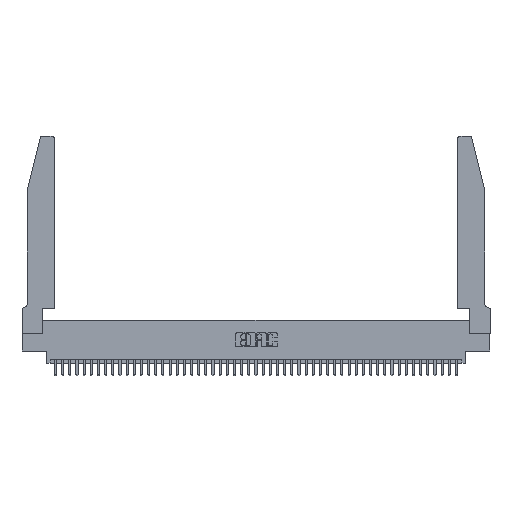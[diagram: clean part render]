
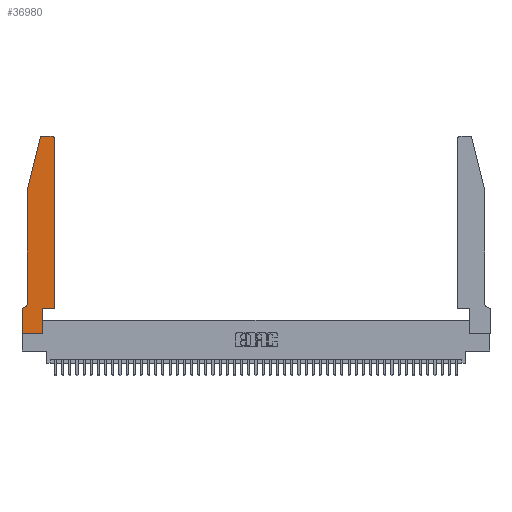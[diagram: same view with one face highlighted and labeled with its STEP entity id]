
A CAD part, top view. The second image highlights one B-rep face of the part: STEP entity #36980.
In plain terms, the highlighted planar face has unit normal (0, 0, 1).
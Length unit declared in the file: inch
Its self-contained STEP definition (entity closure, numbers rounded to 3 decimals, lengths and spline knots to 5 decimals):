
#577 = VERTEX_POINT ( 'NONE', #38761 ) ;
#1104 = EDGE_CURVE ( 'NONE', #37065, #6819, #38696, .T. ) ;
#2470 = ORIENTED_EDGE ( 'NONE', *, *, #8268, .T. ) ;
#2622 = ORIENTED_EDGE ( 'NONE', *, *, #1104, .T. ) ;
#2773 = CARTESIAN_POINT ( 'NONE',  ( 0.25487, 2.72718, 0.37 ) ) ;
#3654 = FACE_OUTER_BOUND ( 'NONE', #13725, .T. ) ;
#4051 = CARTESIAN_POINT ( 'NONE',  ( 0.4505, 2.72, 0.37 ) ) ;
#4359 = PLANE ( 'NONE',  #20301 ) ;
#4523 = CARTESIAN_POINT ( 'NONE',  ( 0., 0.35, 0.37 ) ) ;
#4540 = VERTEX_POINT ( 'NONE', #16303 ) ;
#5442 = CARTESIAN_POINT ( 'NONE',  ( 0., 0., 0.37 ) ) ;
#5513 = LINE ( 'NONE', #27199, #11266 ) ;
#6732 = ORIENTED_EDGE ( 'NONE', *, *, #28557, .T. ) ;
#6754 = ORIENTED_EDGE ( 'NONE', *, *, #29712, .T. ) ;
#6819 = VERTEX_POINT ( 'NONE', #4051 ) ;
#7427 = VECTOR ( 'NONE', #44058, 39.37008 ) ;
#7572 = CARTESIAN_POINT ( 'NONE',  ( 0., 0., 0.37 ) ) ;
#7674 = VECTOR ( 'NONE', #18357, 39.37008 ) ;
#7821 = VECTOR ( 'NONE', #46020, 39.37008 ) ;
#7872 = VECTOR ( 'NONE', #15080, 39.37008 ) ;
#7947 = EDGE_CURVE ( 'NONE', #42472, #577, #43633, .T. ) ;
#8268 = EDGE_CURVE ( 'NONE', #4540, #11509, #31490, .T. ) ;
#8366 = VECTOR ( 'NONE', #32434, 39.37008 ) ;
#8466 = AXIS2_PLACEMENT_3D ( 'NONE', #10056, #24803, #26848 ) ;
#8479 = ORIENTED_EDGE ( 'NONE', *, *, #18645, .T. ) ;
#8747 = CARTESIAN_POINT ( 'NONE',  ( 0.4205, 2.72, 0.37 ) ) ;
#8918 = DIRECTION ( 'NONE',  ( 0., 0., 1. ) ) ;
#9044 = CARTESIAN_POINT ( 'NONE',  ( 0.4505, 0.35, 0.37 ) ) ;
#9473 = CARTESIAN_POINT ( 'NONE',  ( 0.0055, 0.42, 0.37 ) ) ;
#9497 = CARTESIAN_POINT ( 'NONE',  ( 0.2865, 0.35, 0.37 ) ) ;
#9647 = VECTOR ( 'NONE', #31269, 39.37008 ) ;
#9794 = VERTEX_POINT ( 'NONE', #41018 ) ;
#10056 = CARTESIAN_POINT ( 'NONE',  ( 0.284, 2.72, 0.37 ) ) ;
#10927 = EDGE_CURVE ( 'NONE', #577, #16014, #38673, .T. ) ;
#11266 = VECTOR ( 'NONE', #34308, 39.37008 ) ;
#11356 = VERTEX_POINT ( 'NONE', #34246 ) ;
#11509 = VERTEX_POINT ( 'NONE', #7572 ) ;
#11612 = CARTESIAN_POINT ( 'NONE',  ( 0.4205, 2.75, 0.37 ) ) ;
#11989 = LINE ( 'NONE', #15483, #24116 ) ;
#12301 = DIRECTION ( 'NONE',  ( 1., 0., 0. ) ) ;
#12440 = DIRECTION ( 'NONE',  ( 0., 1., 0. ) ) ;
#13406 = CARTESIAN_POINT ( 'NONE',  ( 0.2865, 0.35, 0.37 ) ) ;
#13725 = EDGE_LOOP ( 'NONE', ( #19344, #43618, #42547, #18176, #6732, #8479, #2470, #25183, #6754, #41848, #2622, #16489 ) ) ;
#14187 = VERTEX_POINT ( 'NONE', #32328 ) ;
#14326 = CARTESIAN_POINT ( 'NONE',  ( 0., 0., 0.37 ) ) ;
#15080 = DIRECTION ( 'NONE',  ( -1., 0., 0. ) ) ;
#15483 = CARTESIAN_POINT ( 'NONE',  ( 0.4505, 0.35, 0.37 ) ) ;
#16014 = VERTEX_POINT ( 'NONE', #2773 ) ;
#16086 = LINE ( 'NONE', #25350, #7427 ) ;
#16303 = CARTESIAN_POINT ( 'NONE',  ( 0., 0.35, 0.37 ) ) ;
#16489 = ORIENTED_EDGE ( 'NONE', *, *, #43840, .T. ) ;
#16818 = VECTOR ( 'NONE', #12440, 39.37008 ) ;
#18176 = ORIENTED_EDGE ( 'NONE', *, *, #28774, .T. ) ;
#18357 = DIRECTION ( 'NONE',  ( 1., 0., 0. ) ) ;
#18645 = EDGE_CURVE ( 'NONE', #11356, #4540, #5513, .T. ) ;
#19344 = ORIENTED_EDGE ( 'NONE', *, *, #7947, .T. ) ;
#19802 = EDGE_CURVE ( 'NONE', #16014, #9794, #40128, .T. ) ;
#20301 = AXIS2_PLACEMENT_3D ( 'NONE', #4523, #37547, #30610 ) ;
#23054 = DIRECTION ( 'NONE',  ( 1., 0., 0. ) ) ;
#24058 = EDGE_CURVE ( 'NONE', #45467, #37065, #11989, .T. ) ;
#24116 = VECTOR ( 'NONE', #23054, 39.37008 ) ;
#24803 = DIRECTION ( 'NONE',  ( 0., 0., 1. ) ) ;
#25183 = ORIENTED_EDGE ( 'NONE', *, *, #32283, .T. ) ;
#25350 = CARTESIAN_POINT ( 'NONE',  ( 0.0755, 2., 0.37 ) ) ;
#26848 = DIRECTION ( 'NONE',  ( 1., 0., 0. ) ) ;
#27199 = CARTESIAN_POINT ( 'NONE',  ( 0.0755, 0.35, 0.37 ) ) ;
#27528 = AXIS2_PLACEMENT_3D ( 'NONE', #8747, #8918, #12301 ) ;
#28557 = EDGE_CURVE ( 'NONE', #14187, #11356, #39166, .T. ) ;
#28774 = EDGE_CURVE ( 'NONE', #9794, #14187, #16086, .T. ) ;
#29712 = EDGE_CURVE ( 'NONE', #38966, #45467, #36178, .T. ) ;
#30610 = DIRECTION ( 'NONE',  ( 1., 0., 0. ) ) ;
#31046 = DIRECTION ( 'NONE',  ( 0., 0., -1. ) ) ;
#31269 = DIRECTION ( 'NONE',  ( 0., 1., 0. ) ) ;
#31281 = CARTESIAN_POINT ( 'NONE',  ( 0.4505, 0.35, 0.37 ) ) ;
#31490 = LINE ( 'NONE', #5442, #7821 ) ;
#32283 = EDGE_CURVE ( 'NONE', #11509, #38966, #39449, .T. ) ;
#32328 = CARTESIAN_POINT ( 'NONE',  ( 0.0755, 0.42, 0.37 ) ) ;
#32434 = DIRECTION ( 'NONE',  ( -0.239, -0.971, 0. ) ) ;
#34246 = CARTESIAN_POINT ( 'NONE',  ( 0.0055, 0.35, 0.37 ) ) ;
#34308 = DIRECTION ( 'NONE',  ( -1., 0., 0. ) ) ;
#34810 = CARTESIAN_POINT ( 'NONE',  ( 0.2865, 0., 0.37 ) ) ;
#35246 = DIRECTION ( 'NONE',  ( -1., 0., 0. ) ) ;
#36178 = LINE ( 'NONE', #13406, #9647 ) ;
#36980 = ADVANCED_FACE ( 'NONE', ( #3654 ), #4359, .T. ) ;
#37065 = VERTEX_POINT ( 'NONE', #9044 ) ;
#37547 = DIRECTION ( 'NONE',  ( 0., 0., 1. ) ) ;
#38100 = CIRCLE ( 'NONE', #27528, 0.03 ) ;
#38673 = CIRCLE ( 'NONE', #8466, 0.03 ) ;
#38696 = LINE ( 'NONE', #31281, #16818 ) ;
#38761 = CARTESIAN_POINT ( 'NONE',  ( 0.284, 2.75, 0.37 ) ) ;
#38966 = VERTEX_POINT ( 'NONE', #34810 ) ;
#39166 = CIRCLE ( 'NONE', #44738, 0.07 ) ;
#39449 = LINE ( 'NONE', #14326, #7674 ) ;
#40128 = LINE ( 'NONE', #46605, #8366 ) ;
#41018 = CARTESIAN_POINT ( 'NONE',  ( 0.0755, 2., 0.37 ) ) ;
#41848 = ORIENTED_EDGE ( 'NONE', *, *, #24058, .T. ) ;
#42472 = VERTEX_POINT ( 'NONE', #11612 ) ;
#42547 = ORIENTED_EDGE ( 'NONE', *, *, #19802, .T. ) ;
#43618 = ORIENTED_EDGE ( 'NONE', *, *, #10927, .T. ) ;
#43633 = LINE ( 'NONE', #47690, #7872 ) ;
#43840 = EDGE_CURVE ( 'NONE', #6819, #42472, #38100, .T. ) ;
#44058 = DIRECTION ( 'NONE',  ( 0., -1., 0. ) ) ;
#44738 = AXIS2_PLACEMENT_3D ( 'NONE', #9473, #31046, #35246 ) ;
#45467 = VERTEX_POINT ( 'NONE', #9497 ) ;
#46020 = DIRECTION ( 'NONE',  ( 0., -1., 0. ) ) ;
#46605 = CARTESIAN_POINT ( 'NONE',  ( 0.0755, 2., 0.37 ) ) ;
#47690 = CARTESIAN_POINT ( 'NONE',  ( 0.2605, 2.75, 0.37 ) ) ;
